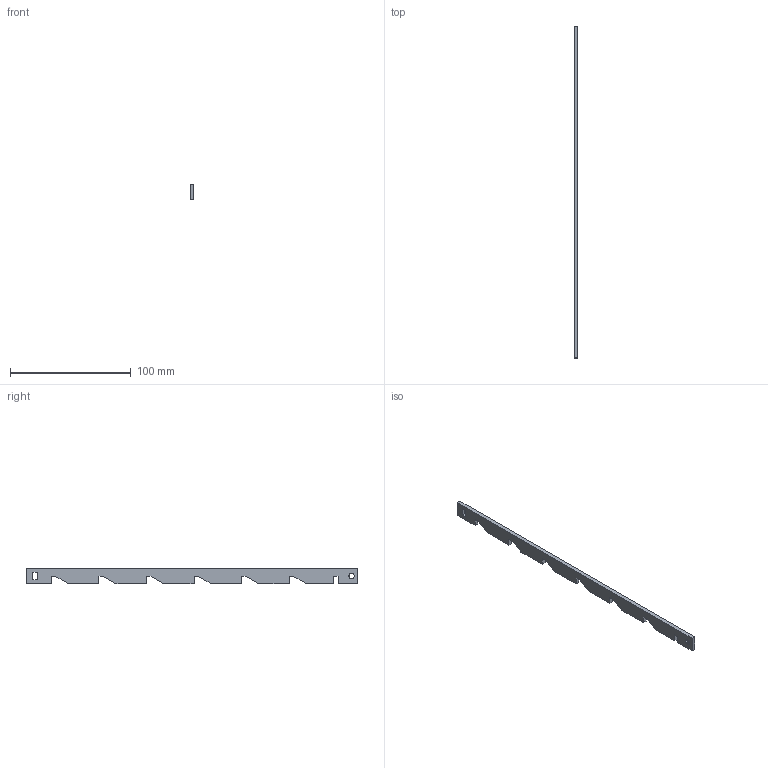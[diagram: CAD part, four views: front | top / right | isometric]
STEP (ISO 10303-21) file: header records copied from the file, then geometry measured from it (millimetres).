
FILE_DESCRIPTION(('FreeCAD Model'),'2;1');
FILE_NAME('Open CASCADE Shape Model','2024-02-27T15:20:58',('Author'),( ''),'Open CASCADE STEP processor 7.5','FreeCAD','Unknown');
FILE_SCHEMA(('AUTOMOTIVE_DESIGN { 1 0 10303 214 1 1 1 1 }'));
Length unit declared in the file: millimetre
Products named in the file (1): LeftTelescopingBar
Bounding box: 3.17 x 275 x 12.7 mm (x, y, z)
Volume: 9839.2 mm3; surface area: 8323.7 mm2
Topology: 1 solids, 1 shells, 40 faces, 113 edges, 75 vertices
Faces by surface type: plane 38, cylinder 1, cone 1
Full cylindrical faces by diameter (mm): 4.5 x1
Entity records: 2771 total; most frequent: CARTESIAN_POINT 455, DIRECTION 424, LINE 334, VECTOR 334, ORIENTED_EDGE 226, PCURVE 226, DEFINITIONAL_REPRESENTATION 226, EDGE_CURVE 113
